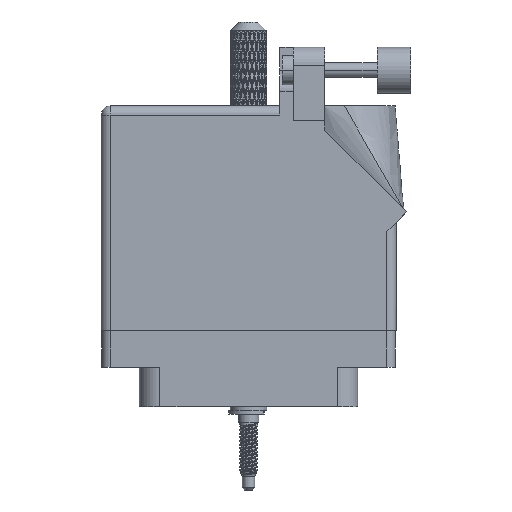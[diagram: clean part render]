
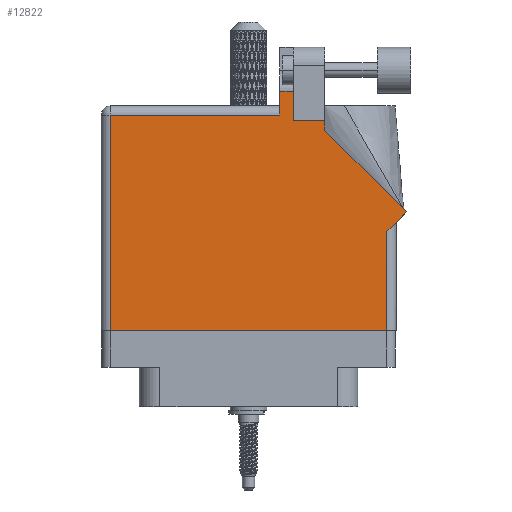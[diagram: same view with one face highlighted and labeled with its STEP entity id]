
A CAD part, front view. The second image highlights one B-rep face of the part: STEP entity #12822.
In plain terms, the highlighted face is planar.
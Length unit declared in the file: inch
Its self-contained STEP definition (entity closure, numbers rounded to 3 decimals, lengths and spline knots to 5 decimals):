
#759 = LINE ( 'NONE', #30854, #103270 ) ;
#1364 = CARTESIAN_POINT ( 'NONE',  ( -0.943, -0.1, 0.455 ) ) ;
#2531 = CARTESIAN_POINT ( 'NONE',  ( 0.212, 1.368, 0.455 ) ) ;
#3565 = CARTESIAN_POINT ( 'NONE',  ( 0.306, 1.5315, 0.455 ) ) ;
#4412 = VECTOR ( 'NONE', #100626, 39.37008 ) ;
#6249 = VERTEX_POINT ( 'NONE', #1364 ) ;
#7447 = CARTESIAN_POINT ( 'NONE',  ( 0.306, 1.33, 0.455 ) ) ;
#8107 = LINE ( 'NONE', #26855, #78663 ) ;
#8538 = DIRECTION ( 'NONE',  ( 0., -1., 0. ) ) ;
#9876 = VERTEX_POINT ( 'NONE', #58032 ) ;
#11617 = LINE ( 'NONE', #27607, #39781 ) ;
#12362 = EDGE_CURVE ( 'NONE', #74498, #29011, #11617, .T. ) ;
#12822 = ADVANCED_FACE ( 'NONE', ( #46296 ), #29877, .F. ) ;
#15772 = VECTOR ( 'NONE', #97749, 39.37008 ) ;
#18510 = LINE ( 'NONE', #83759, #4412 ) ;
#21217 = ORIENTED_EDGE ( 'NONE', *, *, #81833, .T. ) ;
#21235 = ORIENTED_EDGE ( 'NONE', *, *, #90908, .T. ) ;
#22362 = ORIENTED_EDGE ( 'NONE', *, *, #66695, .T. ) ;
#24675 = VECTOR ( 'NONE', #49927, 39.37008 ) ;
#26254 = EDGE_CURVE ( 'NONE', #9876, #102393, #101577, .T. ) ;
#26855 = CARTESIAN_POINT ( 'NONE',  ( 1.005, 0.637, 0.455 ) ) ;
#27607 = CARTESIAN_POINT ( 'NONE',  ( 0.943, 0.637, 0.455 ) ) ;
#29011 = VERTEX_POINT ( 'NONE', #103918 ) ;
#29218 = LINE ( 'NONE', #95265, #44647 ) ;
#29678 = LINE ( 'NONE', #52874, #60364 ) ;
#29877 = PLANE ( 'NONE',  #100715 ) ;
#29895 = VECTOR ( 'NONE', #57579, 39.37008 ) ;
#30854 = CARTESIAN_POINT ( 'NONE',  ( 0.63677, 1.5315, 0.455 ) ) ;
#31603 = ORIENTED_EDGE ( 'NONE', *, *, #12362, .T. ) ;
#32905 = CARTESIAN_POINT ( 'NONE',  ( -1.005, -0.1, 0.455 ) ) ;
#35137 = EDGE_CURVE ( 'NONE', #87583, #42069, #38833, .T. ) ;
#35507 = DIRECTION ( 'NONE',  ( 0.707, 0.707, 0. ) ) ;
#35774 = CARTESIAN_POINT ( 'NONE',  ( 0.943, -0.1, 0.455 ) ) ;
#36542 = EDGE_CURVE ( 'NONE', #101799, #63646, #29678, .T. ) ;
#36938 = DIRECTION ( 'NONE',  ( 0., 1., 0. ) ) ;
#37071 = CARTESIAN_POINT ( 'NONE',  ( -1.005, 1.43, 0.455 ) ) ;
#37435 = DIRECTION ( 'NONE',  ( -1., 0., 0. ) ) ;
#38833 = LINE ( 'NONE', #58176, #24675 ) ;
#39781 = VECTOR ( 'NONE', #36938, 39.37008 ) ;
#39854 = LINE ( 'NONE', #74808, #43665 ) ;
#42069 = VERTEX_POINT ( 'NONE', #2531 ) ;
#42916 = ORIENTED_EDGE ( 'NONE', *, *, #35137, .T. ) ;
#43665 = VECTOR ( 'NONE', #8538, 39.37008 ) ;
#44647 = VECTOR ( 'NONE', #94188, 39.37008 ) ;
#46296 = FACE_OUTER_BOUND ( 'NONE', #46900, .T. ) ;
#46900 = EDGE_LOOP ( 'NONE', ( #105935, #81978, #42916, #21217, #85172, #21235, #31603, #97160, #84372, #22362, #52111 ) ) ;
#49927 = DIRECTION ( 'NONE',  ( 0., -1., 0. ) ) ;
#51654 = LINE ( 'NONE', #82618, #29895 ) ;
#51705 = CARTESIAN_POINT ( 'NONE',  ( 1.07571, 0.70771, 0.455 ) ) ;
#52111 = ORIENTED_EDGE ( 'NONE', *, *, #26254, .T. ) ;
#52874 = CARTESIAN_POINT ( 'NONE',  ( 1.07571, 0.70771, 0.455 ) ) ;
#54700 = CARTESIAN_POINT ( 'NONE',  ( 0.212, 1.5315, 0.455 ) ) ;
#57579 = DIRECTION ( 'NONE',  ( 0., 1., 0. ) ) ;
#58032 = CARTESIAN_POINT ( 'NONE',  ( 0.519, 1.33, 0.455 ) ) ;
#58176 = CARTESIAN_POINT ( 'NONE',  ( 0.212, 1.43, 0.455 ) ) ;
#59362 = LINE ( 'NONE', #32905, #15772 ) ;
#60364 = VECTOR ( 'NONE', #98351, 39.37008 ) ;
#63646 = VERTEX_POINT ( 'NONE', #66006 ) ;
#66006 = CARTESIAN_POINT ( 'NONE',  ( 0.519, 1.26442, 0.455 ) ) ;
#66695 = EDGE_CURVE ( 'NONE', #63646, #9876, #29218, .T. ) ;
#69929 = EDGE_CURVE ( 'NONE', #99077, #87583, #759, .T. ) ;
#74498 = VERTEX_POINT ( 'NONE', #35774 ) ;
#74808 = CARTESIAN_POINT ( 'NONE',  ( -0.943, -0.1, 0.455 ) ) ;
#78663 = VECTOR ( 'NONE', #35507, 39.37008 ) ;
#81246 = VERTEX_POINT ( 'NONE', #92128 ) ;
#81833 = EDGE_CURVE ( 'NONE', #42069, #81246, #18510, .T. ) ;
#81978 = ORIENTED_EDGE ( 'NONE', *, *, #69929, .T. ) ;
#82618 = CARTESIAN_POINT ( 'NONE',  ( 0.306, 1.33, 0.455 ) ) ;
#83759 = CARTESIAN_POINT ( 'NONE',  ( -1.005, 1.368, 0.455 ) ) ;
#84372 = ORIENTED_EDGE ( 'NONE', *, *, #36542, .T. ) ;
#85172 = ORIENTED_EDGE ( 'NONE', *, *, #92984, .T. ) ;
#87583 = VERTEX_POINT ( 'NONE', #54700 ) ;
#88151 = DIRECTION ( 'NONE',  ( -1., 0., 0. ) ) ;
#89195 = EDGE_CURVE ( 'NONE', #29011, #101799, #8107, .T. ) ;
#90908 = EDGE_CURVE ( 'NONE', #6249, #74498, #59362, .T. ) ;
#91083 = EDGE_CURVE ( 'NONE', #102393, #99077, #51654, .T. ) ;
#92128 = CARTESIAN_POINT ( 'NONE',  ( -0.943, 1.368, 0.455 ) ) ;
#92984 = EDGE_CURVE ( 'NONE', #81246, #6249, #39854, .T. ) ;
#94188 = DIRECTION ( 'NONE',  ( 0., 1., 0. ) ) ;
#94330 = DIRECTION ( 'NONE',  ( 0., 0., -1. ) ) ;
#95265 = CARTESIAN_POINT ( 'NONE',  ( 0.519, 1.26442, 0.455 ) ) ;
#96022 = CARTESIAN_POINT ( 'NONE',  ( 0.519, 1.33, 0.455 ) ) ;
#97160 = ORIENTED_EDGE ( 'NONE', *, *, #89195, .T. ) ;
#97749 = DIRECTION ( 'NONE',  ( 1., 0., 0. ) ) ;
#98351 = DIRECTION ( 'NONE',  ( -0.707, 0.707, 0. ) ) ;
#99022 = VECTOR ( 'NONE', #103249, 39.37008 ) ;
#99077 = VERTEX_POINT ( 'NONE', #3565 ) ;
#100626 = DIRECTION ( 'NONE',  ( -1., 0., 0. ) ) ;
#100715 = AXIS2_PLACEMENT_3D ( 'NONE', #37071, #94330, #37435 ) ;
#101577 = LINE ( 'NONE', #96022, #99022 ) ;
#101799 = VERTEX_POINT ( 'NONE', #51705 ) ;
#102393 = VERTEX_POINT ( 'NONE', #7447 ) ;
#103249 = DIRECTION ( 'NONE',  ( -1., 0., 0. ) ) ;
#103270 = VECTOR ( 'NONE', #88151, 39.37008 ) ;
#103918 = CARTESIAN_POINT ( 'NONE',  ( 0.943, 0.575, 0.455 ) ) ;
#105935 = ORIENTED_EDGE ( 'NONE', *, *, #91083, .T. ) ;
